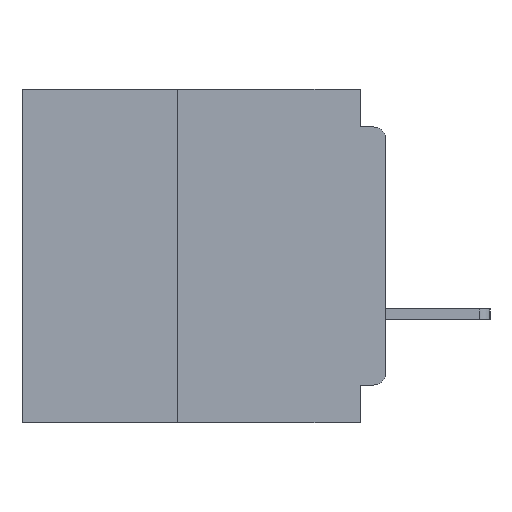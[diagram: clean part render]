
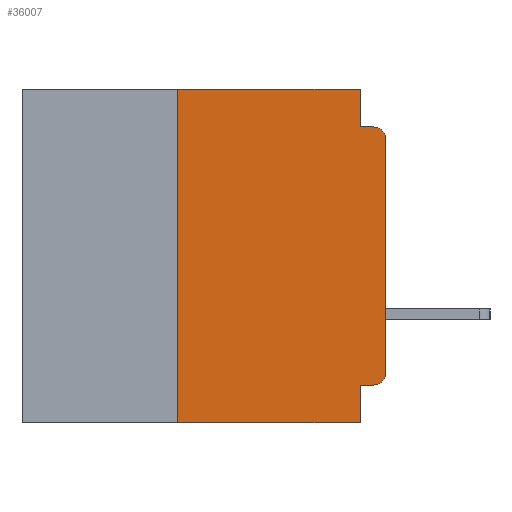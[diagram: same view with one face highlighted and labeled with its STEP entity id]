
A CAD part, left-side view. The second image highlights one B-rep face of the part: STEP entity #36007.
In plain terms, the highlighted planar face has unit normal (-1, 0, 0).
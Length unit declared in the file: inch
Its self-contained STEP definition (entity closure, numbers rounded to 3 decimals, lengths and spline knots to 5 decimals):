
#1588 = CARTESIAN_POINT ( 'NONE',  ( 0., 0.031, -0.355 ) ) ;
#1720 = CARTESIAN_POINT ( 'NONE',  ( 0., 0.031, -0.4 ) ) ;
#2712 = ORIENTED_EDGE ( 'NONE', *, *, #20702, .F. ) ;
#3598 = EDGE_CURVE ( 'NONE', #33225, #28751, #11716, .T. ) ;
#4073 = CARTESIAN_POINT ( 'NONE',  ( 0., 0., 0. ) ) ;
#4509 = CARTESIAN_POINT ( 'NONE',  ( 0., 0.25, 0. ) ) ;
#4672 = CARTESIAN_POINT ( 'NONE',  ( 0., 0., -0.045 ) ) ;
#5203 = FACE_OUTER_BOUND ( 'NONE', #36825, .T. ) ;
#5279 = LINE ( 'NONE', #27295, #43273 ) ;
#6535 = EDGE_CURVE ( 'NONE', #41188, #28751, #44892, .T. ) ;
#6666 = VERTEX_POINT ( 'NONE', #24034 ) ;
#6830 = LINE ( 'NONE', #32065, #44865 ) ;
#6853 = ORIENTED_EDGE ( 'NONE', *, *, #39807, .T. ) ;
#7195 = VECTOR ( 'NONE', #20269, 39.37008 ) ;
#7701 = CARTESIAN_POINT ( 'NONE',  ( 0., 0.031, -0.045 ) ) ;
#9136 = CARTESIAN_POINT ( 'NONE',  ( 0., 0.25, -0.4 ) ) ;
#9753 = VERTEX_POINT ( 'NONE', #33828 ) ;
#10517 = VERTEX_POINT ( 'NONE', #13281 ) ;
#11128 = CARTESIAN_POINT ( 'NONE',  ( 0., 0.015, -0.06 ) ) ;
#11129 = CIRCLE ( 'NONE', #46705, 0.015 ) ;
#11716 = LINE ( 'NONE', #42725, #34808 ) ;
#11947 = ORIENTED_EDGE ( 'NONE', *, *, #6535, .T. ) ;
#13281 = CARTESIAN_POINT ( 'NONE',  ( 0., 0., -0.06 ) ) ;
#14290 = CARTESIAN_POINT ( 'NONE',  ( 0., 0.015, -0.34 ) ) ;
#14809 = DIRECTION ( 'NONE',  ( 0., 0., -1. ) ) ;
#15463 = CARTESIAN_POINT ( 'NONE',  ( 0., 0.015, -0.355 ) ) ;
#15729 = DIRECTION ( 'NONE',  ( 0., -1., 0. ) ) ;
#16924 = LINE ( 'NONE', #9136, #7195 ) ;
#17138 = DIRECTION ( 'NONE',  ( 0., -1., 0. ) ) ;
#17948 = DIRECTION ( 'NONE',  ( 0., 0., -1. ) ) ;
#18031 = DIRECTION ( 'NONE',  ( 1., 0., 0. ) ) ;
#18467 = ORIENTED_EDGE ( 'NONE', *, *, #41639, .F. ) ;
#19944 = CARTESIAN_POINT ( 'NONE',  ( 0., 0., -0.355 ) ) ;
#20269 = DIRECTION ( 'NONE',  ( 0., 0., 1. ) ) ;
#20599 = ORIENTED_EDGE ( 'NONE', *, *, #37474, .F. ) ;
#20693 = LINE ( 'NONE', #4672, #39124 ) ;
#20702 = EDGE_CURVE ( 'NONE', #33085, #33225, #41537, .T. ) ;
#20984 = VERTEX_POINT ( 'NONE', #25280 ) ;
#21969 = VECTOR ( 'NONE', #23704, 39.37008 ) ;
#23657 = AXIS2_PLACEMENT_3D ( 'NONE', #40173, #18031, #43826 ) ;
#23704 = DIRECTION ( 'NONE',  ( 0., 1., 0. ) ) ;
#24034 = CARTESIAN_POINT ( 'NONE',  ( 0., 0., -0.34 ) ) ;
#24114 = CARTESIAN_POINT ( 'NONE',  ( 0., 0.25, -0.4 ) ) ;
#25224 = ORIENTED_EDGE ( 'NONE', *, *, #34592, .F. ) ;
#25280 = CARTESIAN_POINT ( 'NONE',  ( 0., 0.015, -0.045 ) ) ;
#26404 = EDGE_CURVE ( 'NONE', #41621, #9753, #6830, .T. ) ;
#27295 = CARTESIAN_POINT ( 'NONE',  ( 0., 0.031, 0. ) ) ;
#27385 = DIRECTION ( 'NONE',  ( 0., -1., 0. ) ) ;
#27485 = CARTESIAN_POINT ( 'NONE',  ( 0., 0.437, -0.4 ) ) ;
#27826 = LINE ( 'NONE', #4073, #36429 ) ;
#28751 = VERTEX_POINT ( 'NONE', #1720 ) ;
#29129 = VERTEX_POINT ( 'NONE', #7701 ) ;
#32065 = CARTESIAN_POINT ( 'NONE',  ( 0., 0.437, 0. ) ) ;
#33085 = VERTEX_POINT ( 'NONE', #15463 ) ;
#33225 = VERTEX_POINT ( 'NONE', #1588 ) ;
#33828 = CARTESIAN_POINT ( 'NONE',  ( 0., 0.031, 0. ) ) ;
#34592 = EDGE_CURVE ( 'NONE', #9753, #29129, #5279, .T. ) ;
#34808 = VECTOR ( 'NONE', #42634, 39.37008 ) ;
#35135 = VECTOR ( 'NONE', #27385, 39.37008 ) ;
#35636 = AXIS2_PLACEMENT_3D ( 'NONE', #14290, #40088, #17948 ) ;
#36007 = ADVANCED_FACE ( 'NONE', ( #5203 ), #36460, .F. ) ;
#36429 = VECTOR ( 'NONE', #40967, 39.37008 ) ;
#36460 = PLANE ( 'NONE',  #23657 ) ;
#36635 = CIRCLE ( 'NONE', #35636, 0.015 ) ;
#36825 = EDGE_LOOP ( 'NONE', ( #6853, #39189, #18467, #25224, #46431, #20599, #11947, #46418, #2712, #44227 ) ) ;
#36881 = DIRECTION ( 'NONE',  ( -1., 0., 0. ) ) ;
#37080 = EDGE_CURVE ( 'NONE', #33085, #6666, #36635, .T. ) ;
#37474 = EDGE_CURVE ( 'NONE', #41188, #41621, #16924, .T. ) ;
#38369 = DIRECTION ( 'NONE',  ( 0., 0., -1. ) ) ;
#38467 = EDGE_CURVE ( 'NONE', #10517, #20984, #11129, .T. ) ;
#39124 = VECTOR ( 'NONE', #15729, 39.37008 ) ;
#39189 = ORIENTED_EDGE ( 'NONE', *, *, #38467, .T. ) ;
#39807 = EDGE_CURVE ( 'NONE', #6666, #10517, #27826, .T. ) ;
#40088 = DIRECTION ( 'NONE',  ( -1., 0., 0. ) ) ;
#40173 = CARTESIAN_POINT ( 'NONE',  ( 0., 0.437, 0. ) ) ;
#40967 = DIRECTION ( 'NONE',  ( 0., 0., 1. ) ) ;
#41188 = VERTEX_POINT ( 'NONE', #24114 ) ;
#41537 = LINE ( 'NONE', #19944, #21969 ) ;
#41621 = VERTEX_POINT ( 'NONE', #4509 ) ;
#41639 = EDGE_CURVE ( 'NONE', #29129, #20984, #20693, .T. ) ;
#42634 = DIRECTION ( 'NONE',  ( 0., 0., -1. ) ) ;
#42725 = CARTESIAN_POINT ( 'NONE',  ( 0., 0.031, -0.4 ) ) ;
#43273 = VECTOR ( 'NONE', #38369, 39.37008 ) ;
#43826 = DIRECTION ( 'NONE',  ( 0., 0., -1. ) ) ;
#44227 = ORIENTED_EDGE ( 'NONE', *, *, #37080, .T. ) ;
#44865 = VECTOR ( 'NONE', #17138, 39.37008 ) ;
#44892 = LINE ( 'NONE', #27485, #35135 ) ;
#46418 = ORIENTED_EDGE ( 'NONE', *, *, #3598, .F. ) ;
#46431 = ORIENTED_EDGE ( 'NONE', *, *, #26404, .F. ) ;
#46705 = AXIS2_PLACEMENT_3D ( 'NONE', #11128, #36881, #14809 ) ;
